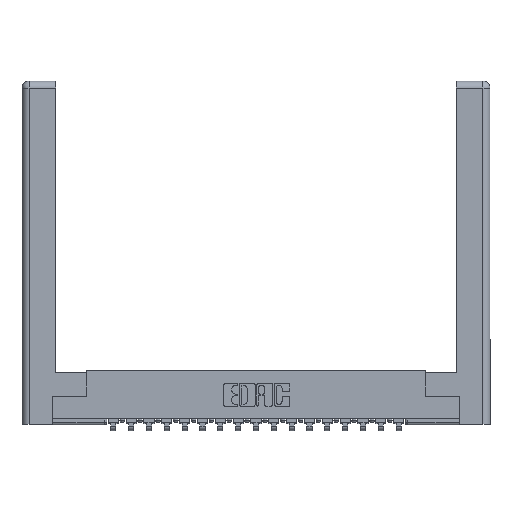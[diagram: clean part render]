
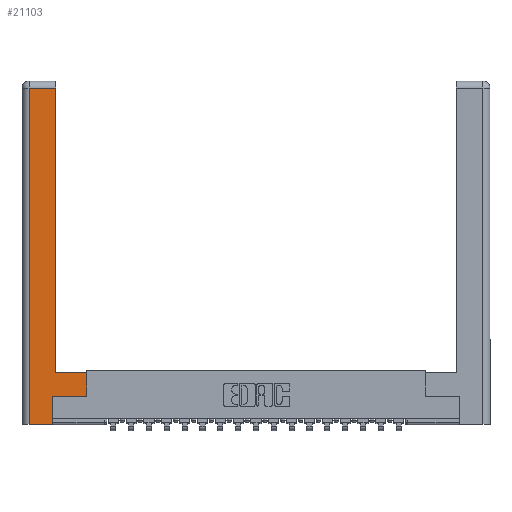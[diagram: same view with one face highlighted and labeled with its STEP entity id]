
A CAD part, top view. The second image highlights one B-rep face of the part: STEP entity #21103.
In plain terms, the highlighted planar face has unit normal (0, 0, 1).
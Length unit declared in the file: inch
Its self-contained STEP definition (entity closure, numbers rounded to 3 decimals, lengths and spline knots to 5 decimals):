
#362 = VERTEX_POINT ( 'NONE', #13361 ) ;
#1058 = VERTEX_POINT ( 'NONE', #10760 ) ;
#1259 = VECTOR ( 'NONE', #1372, 39.37008 ) ;
#1372 = DIRECTION ( 'NONE',  ( 0., -1., 0. ) ) ;
#1391 = ORIENTED_EDGE ( 'NONE', *, *, #18763, .T. ) ;
#1525 = VECTOR ( 'NONE', #2564, 39.37008 ) ;
#1780 = LINE ( 'NONE', #5093, #2860 ) ;
#2361 = CARTESIAN_POINT ( 'NONE',  ( 0.265, 0.245, 0. ) ) ;
#2564 = DIRECTION ( 'NONE',  ( 0., 1., 0. ) ) ;
#2860 = VECTOR ( 'NONE', #11628, 39.37008 ) ;
#3080 = DIRECTION ( 'NONE',  ( 0., 0., -1. ) ) ;
#3897 = ORIENTED_EDGE ( 'NONE', *, *, #17120, .T. ) ;
#4679 = CARTESIAN_POINT ( 'NONE',  ( 0.0615, 0., 0. ) ) ;
#4878 = CARTESIAN_POINT ( 'NONE',  ( 0.565, 0.45, 0. ) ) ;
#4898 = ORIENTED_EDGE ( 'NONE', *, *, #5192, .T. ) ;
#4981 = CARTESIAN_POINT ( 'NONE',  ( 0.565, 0.245, 0. ) ) ;
#5093 = CARTESIAN_POINT ( 'NONE',  ( 0.0615, 2.94, 0. ) ) ;
#5192 = EDGE_CURVE ( 'NONE', #362, #9681, #18817, .T. ) ;
#5230 = VERTEX_POINT ( 'NONE', #7475 ) ;
#5403 = EDGE_CURVE ( 'NONE', #1058, #362, #11214, .T. ) ;
#6498 = CARTESIAN_POINT ( 'NONE',  ( 0.0615, 0., 0. ) ) ;
#7475 = CARTESIAN_POINT ( 'NONE',  ( 0.265, 0., 0. ) ) ;
#7532 = CARTESIAN_POINT ( 'NONE',  ( 0.295, 2.94, 0. ) ) ;
#7673 = CARTESIAN_POINT ( 'NONE',  ( 0.565, 0.45, 0. ) ) ;
#7813 = LINE ( 'NONE', #13047, #14869 ) ;
#7992 = VERTEX_POINT ( 'NONE', #4679 ) ;
#8007 = EDGE_CURVE ( 'NONE', #13904, #10169, #1780, .T. ) ;
#8431 = EDGE_LOOP ( 'NONE', ( #18701, #19543, #1391, #3897, #13035, #12162, #4898, #11736 ) ) ;
#8478 = VECTOR ( 'NONE', #9139, 39.37008 ) ;
#9139 = DIRECTION ( 'NONE',  ( -1., 0., 0. ) ) ;
#9610 = FACE_OUTER_BOUND ( 'NONE', #8431, .T. ) ;
#9681 = VERTEX_POINT ( 'NONE', #4878 ) ;
#10169 = VERTEX_POINT ( 'NONE', #11920 ) ;
#10247 = CARTESIAN_POINT ( 'NONE',  ( 0.295, 0.45, 0. ) ) ;
#10706 = LINE ( 'NONE', #17240, #1525 ) ;
#10707 = EDGE_CURVE ( 'NONE', #19017, #13904, #10706, .T. ) ;
#10760 = CARTESIAN_POINT ( 'NONE',  ( 0.265, 0.245, 0. ) ) ;
#11214 = LINE ( 'NONE', #4981, #16478 ) ;
#11353 = VECTOR ( 'NONE', #14892, 39.37008 ) ;
#11409 = DIRECTION ( 'NONE',  ( 1., 0., 0. ) ) ;
#11532 = DIRECTION ( 'NONE',  ( -1., 0., 0. ) ) ;
#11628 = DIRECTION ( 'NONE',  ( -1., 0., 0. ) ) ;
#11736 = ORIENTED_EDGE ( 'NONE', *, *, #20459, .T. ) ;
#11799 = EDGE_CURVE ( 'NONE', #5230, #1058, #12001, .T. ) ;
#11920 = CARTESIAN_POINT ( 'NONE',  ( 0.0615, 2.94, 0. ) ) ;
#12001 = LINE ( 'NONE', #2361, #11353 ) ;
#12028 = LINE ( 'NONE', #15556, #8478 ) ;
#12162 = ORIENTED_EDGE ( 'NONE', *, *, #5403, .T. ) ;
#12935 = CARTESIAN_POINT ( 'NONE',  ( 0., 0., 0. ) ) ;
#12950 = DIRECTION ( 'NONE',  ( 1., 0., 0. ) ) ;
#13035 = ORIENTED_EDGE ( 'NONE', *, *, #11799, .T. ) ;
#13047 = CARTESIAN_POINT ( 'NONE',  ( 0.265, 0., 0. ) ) ;
#13296 = AXIS2_PLACEMENT_3D ( 'NONE', #12935, #3080, #11532 ) ;
#13361 = CARTESIAN_POINT ( 'NONE',  ( 0.565, 0.245, 0. ) ) ;
#13904 = VERTEX_POINT ( 'NONE', #7532 ) ;
#14869 = VECTOR ( 'NONE', #12950, 39.37008 ) ;
#14892 = DIRECTION ( 'NONE',  ( 0., 1., 0. ) ) ;
#15556 = CARTESIAN_POINT ( 'NONE',  ( 0.295, 0.45, 0. ) ) ;
#16478 = VECTOR ( 'NONE', #11409, 39.37008 ) ;
#17120 = EDGE_CURVE ( 'NONE', #7992, #5230, #7813, .T. ) ;
#17240 = CARTESIAN_POINT ( 'NONE',  ( 0.295, 3., 0. ) ) ;
#17953 = LINE ( 'NONE', #6498, #1259 ) ;
#18701 = ORIENTED_EDGE ( 'NONE', *, *, #10707, .T. ) ;
#18763 = EDGE_CURVE ( 'NONE', #10169, #7992, #17953, .T. ) ;
#18817 = LINE ( 'NONE', #7673, #19196 ) ;
#19017 = VERTEX_POINT ( 'NONE', #10247 ) ;
#19196 = VECTOR ( 'NONE', #20619, 39.37008 ) ;
#19339 = PLANE ( 'NONE',  #13296 ) ;
#19543 = ORIENTED_EDGE ( 'NONE', *, *, #8007, .T. ) ;
#20459 = EDGE_CURVE ( 'NONE', #9681, #19017, #12028, .T. ) ;
#20619 = DIRECTION ( 'NONE',  ( 0., 1., 0. ) ) ;
#21103 = ADVANCED_FACE ( 'NONE', ( #9610 ), #19339, .F. ) ;
